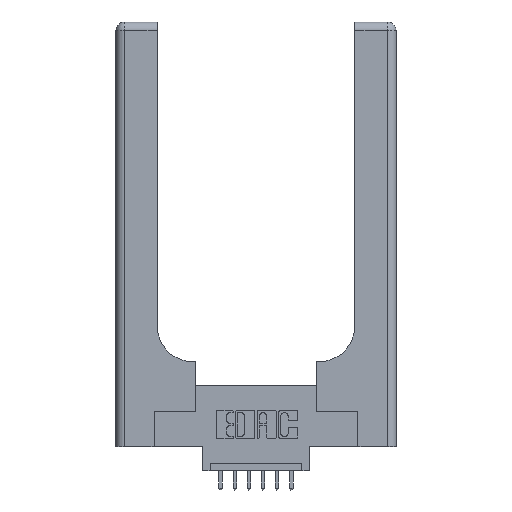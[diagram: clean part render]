
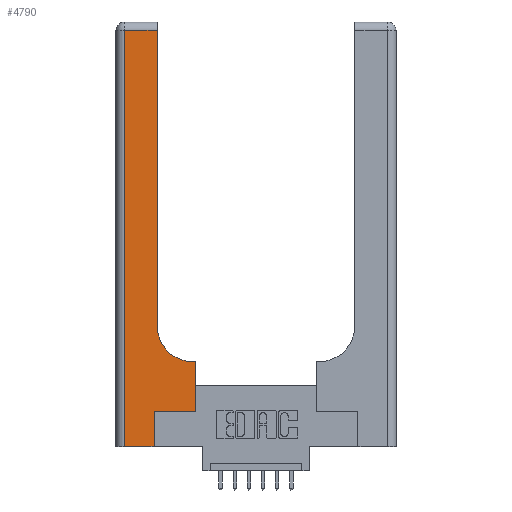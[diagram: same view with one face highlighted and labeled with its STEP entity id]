
A CAD part, top view. The second image highlights one B-rep face of the part: STEP entity #4790.
In plain terms, the highlighted planar face has unit normal (0, 0, 1).
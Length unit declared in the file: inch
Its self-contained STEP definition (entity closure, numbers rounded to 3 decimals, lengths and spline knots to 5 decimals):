
#269 = CARTESIAN_POINT ( 'NONE',  ( 0., 3., 0.37 ) ) ;
#369 = EDGE_CURVE ( 'NONE', #14486, #12952, #7939, .T. ) ;
#575 = VECTOR ( 'NONE', #5864, 39.37008 ) ;
#958 = AXIS2_PLACEMENT_3D ( 'NONE', #269, #8245, #12803 ) ;
#993 = VERTEX_POINT ( 'NONE', #3996 ) ;
#1163 = CARTESIAN_POINT ( 'NONE',  ( 0.5415, 0.6, 0.37 ) ) ;
#1600 = DIRECTION ( 'NONE',  ( 1., 0., 0. ) ) ;
#1637 = VERTEX_POINT ( 'NONE', #3587 ) ;
#1682 = ORIENTED_EDGE ( 'NONE', *, *, #369, .T. ) ;
#1865 = VECTOR ( 'NONE', #1600, 39.37008 ) ;
#1874 = CARTESIAN_POINT ( 'NONE',  ( 0.269, 0., 0.37 ) ) ;
#2126 = DIRECTION ( 'NONE',  ( 0., 1., 0. ) ) ;
#2132 = CARTESIAN_POINT ( 'NONE',  ( 0., 0., 0.37 ) ) ;
#2279 = LINE ( 'NONE', #7732, #7442 ) ;
#2439 = VECTOR ( 'NONE', #6519, 39.37008 ) ;
#2455 = CARTESIAN_POINT ( 'NONE',  ( 0.2915, 0.6, 0.37 ) ) ;
#3581 = CARTESIAN_POINT ( 'NONE',  ( 0.5585, 0.25, 0.37 ) ) ;
#3587 = CARTESIAN_POINT ( 'NONE',  ( 0.2915, 0.85, 0.37 ) ) ;
#3686 = PLANE ( 'NONE',  #958 ) ;
#3930 = ORIENTED_EDGE ( 'NONE', *, *, #12227, .T. ) ;
#3993 = LINE ( 'NONE', #8941, #8252 ) ;
#3996 = CARTESIAN_POINT ( 'NONE',  ( 0.06, 2.94, 0.37 ) ) ;
#4373 = VECTOR ( 'NONE', #13499, 39.37008 ) ;
#4463 = VERTEX_POINT ( 'NONE', #10054 ) ;
#4504 = DIRECTION ( 'NONE',  ( 0., 1., 0. ) ) ;
#4588 = EDGE_CURVE ( 'NONE', #12952, #4463, #14567, .T. ) ;
#4663 = FACE_OUTER_BOUND ( 'NONE', #11903, .T. ) ;
#4790 = ADVANCED_FACE ( 'NONE', ( #4663 ), #3686, .F. ) ;
#5143 = CARTESIAN_POINT ( 'NONE',  ( 0.06, 0., 0.37 ) ) ;
#5669 = CARTESIAN_POINT ( 'NONE',  ( 0., 2.94, 0.37 ) ) ;
#5697 = VERTEX_POINT ( 'NONE', #5143 ) ;
#5848 = ORIENTED_EDGE ( 'NONE', *, *, #6777, .T. ) ;
#5864 = DIRECTION ( 'NONE',  ( -1., 0., 0. ) ) ;
#5908 = ORIENTED_EDGE ( 'NONE', *, *, #11704, .T. ) ;
#6265 = EDGE_CURVE ( 'NONE', #1637, #13103, #2279, .T. ) ;
#6300 = VERTEX_POINT ( 'NONE', #1874 ) ;
#6519 = DIRECTION ( 'NONE',  ( 1., 0., 0. ) ) ;
#6622 = DIRECTION ( 'NONE',  ( 1., 0., 0. ) ) ;
#6777 = EDGE_CURVE ( 'NONE', #5697, #6300, #10275, .T. ) ;
#6976 = CARTESIAN_POINT ( 'NONE',  ( 0.5585, 0.25, 0.37 ) ) ;
#7046 = LINE ( 'NONE', #10303, #4373 ) ;
#7157 = VECTOR ( 'NONE', #12652, 39.37008 ) ;
#7442 = VECTOR ( 'NONE', #4504, 39.37008 ) ;
#7732 = CARTESIAN_POINT ( 'NONE',  ( 0.2915, 3., 0.37 ) ) ;
#7939 = LINE ( 'NONE', #13677, #1865 ) ;
#8245 = DIRECTION ( 'NONE',  ( 0., 0., -1. ) ) ;
#8252 = VECTOR ( 'NONE', #2126, 39.37008 ) ;
#8281 = DIRECTION ( 'NONE',  ( -1., 0., 0. ) ) ;
#8371 = EDGE_CURVE ( 'NONE', #4463, #10546, #12703, .T. ) ;
#8915 = ORIENTED_EDGE ( 'NONE', *, *, #9835, .T. ) ;
#8941 = CARTESIAN_POINT ( 'NONE',  ( 0.269, 0., 0.37 ) ) ;
#9835 = EDGE_CURVE ( 'NONE', #10546, #1637, #9951, .T. ) ;
#9951 = CIRCLE ( 'NONE', #12163, 0.25 ) ;
#10054 = CARTESIAN_POINT ( 'NONE',  ( 0.5585, 0.6, 0.37 ) ) ;
#10062 = VECTOR ( 'NONE', #8281, 39.37008 ) ;
#10275 = LINE ( 'NONE', #2132, #2439 ) ;
#10303 = CARTESIAN_POINT ( 'NONE',  ( 0.06, 3., 0.37 ) ) ;
#10546 = VERTEX_POINT ( 'NONE', #1163 ) ;
#11095 = LINE ( 'NONE', #5669, #575 ) ;
#11503 = CARTESIAN_POINT ( 'NONE',  ( 0.5415, 0.85, 0.37 ) ) ;
#11514 = ORIENTED_EDGE ( 'NONE', *, *, #8371, .T. ) ;
#11613 = CARTESIAN_POINT ( 'NONE',  ( 0.2915, 2.94, 0.37 ) ) ;
#11704 = EDGE_CURVE ( 'NONE', #993, #5697, #7046, .T. ) ;
#11903 = EDGE_LOOP ( 'NONE', ( #12339, #3930, #5908, #5848, #14243, #1682, #11957, #11514, #8915 ) ) ;
#11957 = ORIENTED_EDGE ( 'NONE', *, *, #4588, .T. ) ;
#12112 = EDGE_CURVE ( 'NONE', #6300, #14486, #3993, .T. ) ;
#12163 = AXIS2_PLACEMENT_3D ( 'NONE', #11503, #12433, #6622 ) ;
#12227 = EDGE_CURVE ( 'NONE', #13103, #993, #11095, .T. ) ;
#12339 = ORIENTED_EDGE ( 'NONE', *, *, #6265, .T. ) ;
#12433 = DIRECTION ( 'NONE',  ( 0., 0., -1. ) ) ;
#12652 = DIRECTION ( 'NONE',  ( 0., 1., 0. ) ) ;
#12703 = LINE ( 'NONE', #2455, #10062 ) ;
#12803 = DIRECTION ( 'NONE',  ( -1., 0., 0. ) ) ;
#12952 = VERTEX_POINT ( 'NONE', #6976 ) ;
#13103 = VERTEX_POINT ( 'NONE', #11613 ) ;
#13159 = CARTESIAN_POINT ( 'NONE',  ( 0.269, 0.25, 0.37 ) ) ;
#13499 = DIRECTION ( 'NONE',  ( 0., -1., 0. ) ) ;
#13677 = CARTESIAN_POINT ( 'NONE',  ( 0.269, 0.25, 0.37 ) ) ;
#14243 = ORIENTED_EDGE ( 'NONE', *, *, #12112, .T. ) ;
#14486 = VERTEX_POINT ( 'NONE', #13159 ) ;
#14567 = LINE ( 'NONE', #3581, #7157 ) ;
